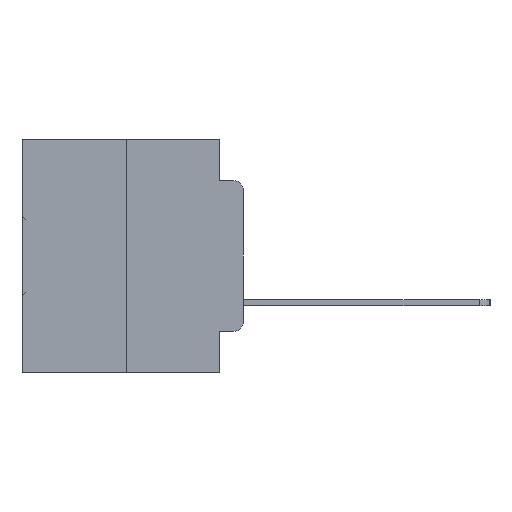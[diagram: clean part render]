
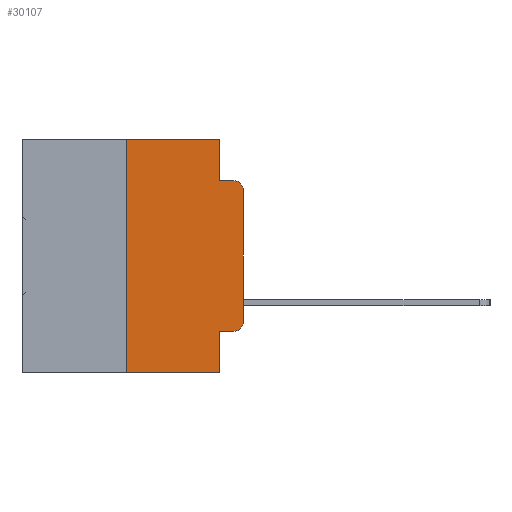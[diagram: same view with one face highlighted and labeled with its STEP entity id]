
A CAD part, left-side view. The second image highlights one B-rep face of the part: STEP entity #30107.
In plain terms, the highlighted planar face has unit normal (-1, 0, 0).
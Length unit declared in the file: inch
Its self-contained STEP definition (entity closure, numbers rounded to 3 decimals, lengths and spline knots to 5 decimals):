
#417 = VECTOR ( 'NONE', #21435, 39.37008 ) ;
#451 = VERTEX_POINT ( 'NONE', #28618 ) ;
#493 = VERTEX_POINT ( 'NONE', #25958 ) ;
#725 = ORIENTED_EDGE ( 'NONE', *, *, #11888, .F. ) ;
#839 = DIRECTION ( 'NONE',  ( 0., 0., 1. ) ) ;
#1642 = EDGE_CURVE ( 'NONE', #31195, #5470, #25879, .T. ) ;
#2935 = VERTEX_POINT ( 'NONE', #18200 ) ;
#3152 = ORIENTED_EDGE ( 'NONE', *, *, #31141, .T. ) ;
#3400 = EDGE_CURVE ( 'NONE', #31195, #23627, #27310, .T. ) ;
#3790 = CARTESIAN_POINT ( 'NONE',  ( 0., 0.473, -0.5 ) ) ;
#4744 = CARTESIAN_POINT ( 'NONE',  ( 0., 0.051, -0.0885 ) ) ;
#5116 = DIRECTION ( 'NONE',  ( 0., -1., 0. ) ) ;
#5316 = CARTESIAN_POINT ( 'NONE',  ( 0., 0.02, -0.4115 ) ) ;
#5470 = VERTEX_POINT ( 'NONE', #5316 ) ;
#6170 = AXIS2_PLACEMENT_3D ( 'NONE', #6488, #24209, #9010 ) ;
#6324 = VECTOR ( 'NONE', #6614, 39.37008 ) ;
#6488 = CARTESIAN_POINT ( 'NONE',  ( 0., 0.02, -0.1085 ) ) ;
#6614 = DIRECTION ( 'NONE',  ( 0., 0., -1. ) ) ;
#6805 = EDGE_CURVE ( 'NONE', #7733, #451, #15720, .T. ) ;
#6858 = VECTOR ( 'NONE', #24371, 39.37008 ) ;
#6912 = EDGE_CURVE ( 'NONE', #7733, #23627, #26726, .T. ) ;
#7733 = VERTEX_POINT ( 'NONE', #22511 ) ;
#8900 = VECTOR ( 'NONE', #839, 39.37008 ) ;
#9010 = DIRECTION ( 'NONE',  ( 0., 0., -1. ) ) ;
#9082 = CARTESIAN_POINT ( 'NONE',  ( 0., 0.051, 0. ) ) ;
#9274 = VERTEX_POINT ( 'NONE', #28671 ) ;
#10214 = CARTESIAN_POINT ( 'NONE',  ( 0., 0.473, 0. ) ) ;
#10262 = CARTESIAN_POINT ( 'NONE',  ( 0., 0., -0.1085 ) ) ;
#11042 = FACE_OUTER_BOUND ( 'NONE', #25933, .T. ) ;
#11352 = DIRECTION ( 'NONE',  ( 0., 0., 1. ) ) ;
#11888 = EDGE_CURVE ( 'NONE', #26588, #2935, #13615, .T. ) ;
#11945 = CARTESIAN_POINT ( 'NONE',  ( 0., 0.02, -0.3915 ) ) ;
#12388 = DIRECTION ( 'NONE',  ( 0., -1., 0. ) ) ;
#12481 = VECTOR ( 'NONE', #26597, 39.37008 ) ;
#12959 = LINE ( 'NONE', #29018, #19728 ) ;
#13261 = AXIS2_PLACEMENT_3D ( 'NONE', #11945, #29623, #14534 ) ;
#13615 = LINE ( 'NONE', #19322, #6858 ) ;
#13866 = CARTESIAN_POINT ( 'NONE',  ( 0., 0.473, 0. ) ) ;
#14534 = DIRECTION ( 'NONE',  ( 0., 0., -1. ) ) ;
#15357 = EDGE_CURVE ( 'NONE', #2935, #493, #29159, .T. ) ;
#15520 = ORIENTED_EDGE ( 'NONE', *, *, #23063, .F. ) ;
#15720 = LINE ( 'NONE', #23656, #8900 ) ;
#15794 = VECTOR ( 'NONE', #12388, 39.37008 ) ;
#16438 = DIRECTION ( 'NONE',  ( 0., 0., -1. ) ) ;
#17035 = EDGE_CURVE ( 'NONE', #28708, #493, #31379, .T. ) ;
#17770 = ORIENTED_EDGE ( 'NONE', *, *, #6805, .F. ) ;
#18200 = CARTESIAN_POINT ( 'NONE',  ( 0., 0.051, -0.0885 ) ) ;
#18235 = ORIENTED_EDGE ( 'NONE', *, *, #20447, .T. ) ;
#18737 = VECTOR ( 'NONE', #5116, 39.37008 ) ;
#19057 = ORIENTED_EDGE ( 'NONE', *, *, #3400, .F. ) ;
#19322 = CARTESIAN_POINT ( 'NONE',  ( 0., 0.051, 0. ) ) ;
#19496 = CARTESIAN_POINT ( 'NONE',  ( 0., 0.051, 0. ) ) ;
#19728 = VECTOR ( 'NONE', #11352, 39.37008 ) ;
#20326 = CARTESIAN_POINT ( 'NONE',  ( 0., 0.051, -0.5 ) ) ;
#20447 = EDGE_CURVE ( 'NONE', #9274, #28708, #12959, .T. ) ;
#21435 = DIRECTION ( 'NONE',  ( 0., -1., 0. ) ) ;
#22511 = CARTESIAN_POINT ( 'NONE',  ( 0., 0.25, -0.5 ) ) ;
#23063 = EDGE_CURVE ( 'NONE', #451, #26588, #25455, .T. ) ;
#23627 = VERTEX_POINT ( 'NONE', #20326 ) ;
#23656 = CARTESIAN_POINT ( 'NONE',  ( 0., 0.25, 0. ) ) ;
#24209 = DIRECTION ( 'NONE',  ( -1., 0., 0. ) ) ;
#24371 = DIRECTION ( 'NONE',  ( 0., 0., -1. ) ) ;
#25455 = LINE ( 'NONE', #10214, #18737 ) ;
#25879 = LINE ( 'NONE', #31683, #417 ) ;
#25933 = EDGE_LOOP ( 'NONE', ( #18235, #30615, #32059, #725, #15520, #17770, #26897, #19057, #28370, #3152 ) ) ;
#25958 = CARTESIAN_POINT ( 'NONE',  ( 0., 0.02, -0.0885 ) ) ;
#26449 = PLANE ( 'NONE',  #29303 ) ;
#26588 = VERTEX_POINT ( 'NONE', #9082 ) ;
#26597 = DIRECTION ( 'NONE',  ( 0., -1., 0. ) ) ;
#26726 = LINE ( 'NONE', #3790, #12481 ) ;
#26897 = ORIENTED_EDGE ( 'NONE', *, *, #6912, .T. ) ;
#27104 = CARTESIAN_POINT ( 'NONE',  ( 0., 0.051, -0.4115 ) ) ;
#27310 = LINE ( 'NONE', #19496, #6324 ) ;
#28370 = ORIENTED_EDGE ( 'NONE', *, *, #1642, .T. ) ;
#28618 = CARTESIAN_POINT ( 'NONE',  ( 0., 0.25, 0. ) ) ;
#28671 = CARTESIAN_POINT ( 'NONE',  ( 0., 0., -0.3915 ) ) ;
#28708 = VERTEX_POINT ( 'NONE', #10262 ) ;
#28808 = CIRCLE ( 'NONE', #13261, 0.02 ) ;
#29018 = CARTESIAN_POINT ( 'NONE',  ( 0., 0., 0. ) ) ;
#29159 = LINE ( 'NONE', #4744, #15794 ) ;
#29303 = AXIS2_PLACEMENT_3D ( 'NONE', #13866, #31473, #16438 ) ;
#29623 = DIRECTION ( 'NONE',  ( -1., 0., 0. ) ) ;
#30107 = ADVANCED_FACE ( 'NONE', ( #11042 ), #26449, .F. ) ;
#30615 = ORIENTED_EDGE ( 'NONE', *, *, #17035, .T. ) ;
#31141 = EDGE_CURVE ( 'NONE', #5470, #9274, #28808, .T. ) ;
#31195 = VERTEX_POINT ( 'NONE', #27104 ) ;
#31379 = CIRCLE ( 'NONE', #6170, 0.02 ) ;
#31473 = DIRECTION ( 'NONE',  ( 1., 0., 0. ) ) ;
#31683 = CARTESIAN_POINT ( 'NONE',  ( 0., 0.051, -0.4115 ) ) ;
#32059 = ORIENTED_EDGE ( 'NONE', *, *, #15357, .F. ) ;
